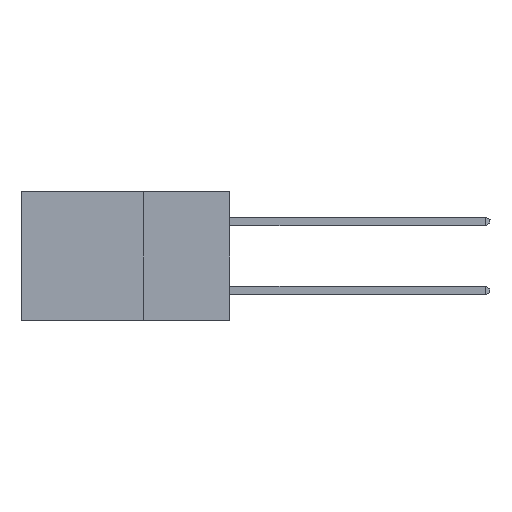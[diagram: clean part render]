
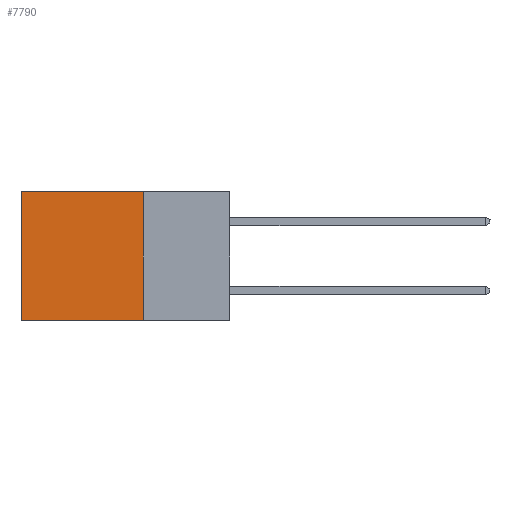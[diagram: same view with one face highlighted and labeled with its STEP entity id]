
A CAD part, left-side view. The second image highlights one B-rep face of the part: STEP entity #7790.
In plain terms, the highlighted planar face has unit normal (-1, 0, 0).
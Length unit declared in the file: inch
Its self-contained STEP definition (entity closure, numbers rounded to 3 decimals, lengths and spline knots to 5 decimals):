
#668 = VERTEX_POINT ( 'NONE', #9224 ) ;
#1153 = VECTOR ( 'NONE', #12901, 39.37008 ) ;
#1723 = LINE ( 'NONE', #8695, #16252 ) ;
#2778 = DIRECTION ( 'NONE',  ( 0., 1., 0. ) ) ;
#2863 = EDGE_CURVE ( 'NONE', #8676, #4891, #11619, .T. ) ;
#3530 = VECTOR ( 'NONE', #2778, 39.37008 ) ;
#3760 = CARTESIAN_POINT ( 'NONE',  ( 0.2615, 0.25, -0.37 ) ) ;
#4151 = ORIENTED_EDGE ( 'NONE', *, *, #15261, .F. ) ;
#4677 = ORIENTED_EDGE ( 'NONE', *, *, #13561, .T. ) ;
#4891 = VERTEX_POINT ( 'NONE', #6774 ) ;
#5224 = FACE_OUTER_BOUND ( 'NONE', #17672, .T. ) ;
#5840 = LINE ( 'NONE', #9840, #3530 ) ;
#5961 = AXIS2_PLACEMENT_3D ( 'NONE', #13531, #16131, #6428 ) ;
#6110 = ORIENTED_EDGE ( 'NONE', *, *, #2863, .F. ) ;
#6428 = DIRECTION ( 'NONE',  ( 0., 0., -1. ) ) ;
#6703 = ORIENTED_EDGE ( 'NONE', *, *, #14103, .T. ) ;
#6774 = CARTESIAN_POINT ( 'NONE',  ( 0.2615, 0.6, -0.37 ) ) ;
#7380 = VECTOR ( 'NONE', #13487, 39.37008 ) ;
#7790 = ADVANCED_FACE ( 'NONE', ( #5224 ), #17611, .F. ) ;
#8676 = VERTEX_POINT ( 'NONE', #10449 ) ;
#8695 = CARTESIAN_POINT ( 'NONE',  ( 0.2615, 0.6, -0.37 ) ) ;
#8918 = VERTEX_POINT ( 'NONE', #13932 ) ;
#9224 = CARTESIAN_POINT ( 'NONE',  ( 0.2615, 0.6, 0. ) ) ;
#9840 = CARTESIAN_POINT ( 'NONE',  ( 0.2615, 0.25, 0. ) ) ;
#10449 = CARTESIAN_POINT ( 'NONE',  ( 0.2615, 0.25, -0.37 ) ) ;
#11619 = LINE ( 'NONE', #13088, #1153 ) ;
#12282 = LINE ( 'NONE', #3760, #7380 ) ;
#12901 = DIRECTION ( 'NONE',  ( 0., 1., 0. ) ) ;
#13026 = DIRECTION ( 'NONE',  ( 0., 0., -1. ) ) ;
#13088 = CARTESIAN_POINT ( 'NONE',  ( 0.2615, 0.25, -0.37 ) ) ;
#13487 = DIRECTION ( 'NONE',  ( 0., 0., -1. ) ) ;
#13531 = CARTESIAN_POINT ( 'NONE',  ( 0.2615, 0.25, -0.37 ) ) ;
#13561 = EDGE_CURVE ( 'NONE', #8918, #668, #5840, .T. ) ;
#13932 = CARTESIAN_POINT ( 'NONE',  ( 0.2615, 0.25, 0. ) ) ;
#14103 = EDGE_CURVE ( 'NONE', #668, #4891, #1723, .T. ) ;
#15261 = EDGE_CURVE ( 'NONE', #8918, #8676, #12282, .T. ) ;
#16131 = DIRECTION ( 'NONE',  ( 1., 0., 0. ) ) ;
#16252 = VECTOR ( 'NONE', #13026, 39.37008 ) ;
#17611 = PLANE ( 'NONE',  #5961 ) ;
#17672 = EDGE_LOOP ( 'NONE', ( #6703, #6110, #4151, #4677 ) ) ;
